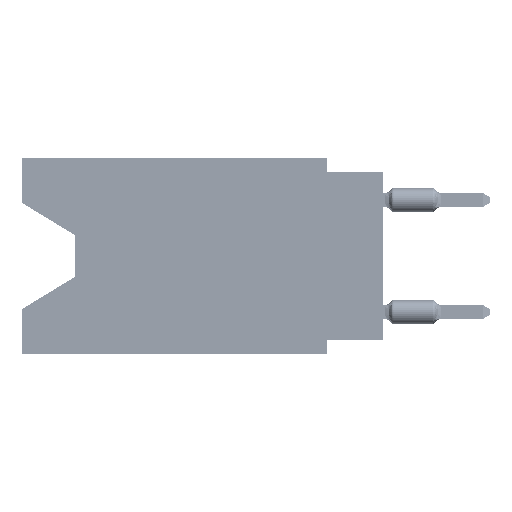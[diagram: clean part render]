
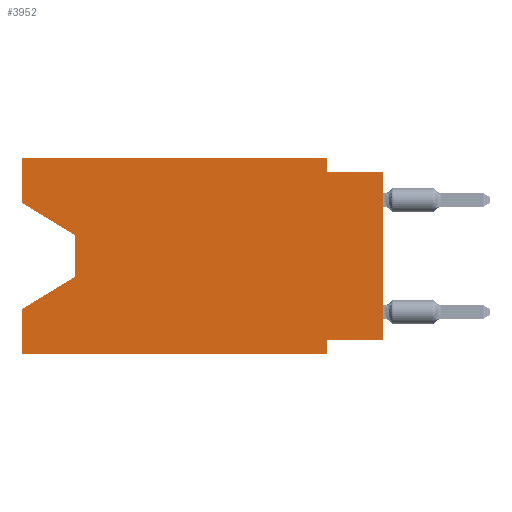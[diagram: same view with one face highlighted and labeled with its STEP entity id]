
A CAD part, left-side view. The second image highlights one B-rep face of the part: STEP entity #3952.
In plain terms, the highlighted planar face has unit normal (-1, 0, 0).
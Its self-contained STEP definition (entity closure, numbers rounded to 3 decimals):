
#749 = DIRECTION ( 'NONE',  ( 0., 0., 1. ) ) ;
#842 = VECTOR ( 'NONE', #63957, 1000. ) ;
#1870 = ORIENTED_EDGE ( 'NONE', *, *, #36977, .F. ) ;
#2698 = LINE ( 'NONE', #42277, #842 ) ;
#2990 = VECTOR ( 'NONE', #46452, 1000. ) ;
#3332 = VECTOR ( 'NONE', #9273, 1000. ) ;
#3509 = CARTESIAN_POINT ( 'NONE',  ( 0., 0., 0. ) ) ;
#3927 = EDGE_CURVE ( 'NONE', #44128, #29172, #12107, .T. ) ;
#3952 = ADVANCED_FACE ( 'NONE', ( #28903 ), #52056, .F. ) ;
#4749 = EDGE_CURVE ( 'NONE', #51776, #22948, #20185, .T. ) ;
#5682 = ORIENTED_EDGE ( 'NONE', *, *, #47351, .F. ) ;
#6222 = ORIENTED_EDGE ( 'NONE', *, *, #25716, .T. ) ;
#6600 = ORIENTED_EDGE ( 'NONE', *, *, #39897, .F. ) ;
#6983 = DIRECTION ( 'NONE',  ( 0., 1., 0. ) ) ;
#7105 = CARTESIAN_POINT ( 'NONE',  ( 0., 16.383, 0. ) ) ;
#7772 = VERTEX_POINT ( 'NONE', #64254 ) ;
#8877 = EDGE_CURVE ( 'NONE', #12186, #42481, #66267, .T. ) ;
#9273 = DIRECTION ( 'NONE',  ( 0., -0.855, -0.519 ) ) ;
#9658 = ORIENTED_EDGE ( 'NONE', *, *, #40314, .F. ) ;
#10961 = CARTESIAN_POINT ( 'NONE',  ( 0., 2.54, -0.635 ) ) ;
#11865 = DIRECTION ( 'NONE',  ( 0., -1., 0. ) ) ;
#12107 = LINE ( 'NONE', #68491, #2990 ) ;
#12186 = VERTEX_POINT ( 'NONE', #27859 ) ;
#12987 = VECTOR ( 'NONE', #15011, 1000. ) ;
#14540 = LINE ( 'NONE', #60436, #3332 ) ;
#15011 = DIRECTION ( 'NONE',  ( 0., 0., -1. ) ) ;
#15600 = ORIENTED_EDGE ( 'NONE', *, *, #35275, .T. ) ;
#17604 = CARTESIAN_POINT ( 'NONE',  ( 0., 13.97, -5.385 ) ) ;
#18115 = VECTOR ( 'NONE', #22621, 1000. ) ;
#18387 = CARTESIAN_POINT ( 'NONE',  ( 0., 0., -8.255 ) ) ;
#20185 = LINE ( 'NONE', #68590, #36137 ) ;
#20604 = CARTESIAN_POINT ( 'NONE',  ( 0., 13.97, -3.505 ) ) ;
#21716 = LINE ( 'NONE', #20604, #12987 ) ;
#22621 = DIRECTION ( 'NONE',  ( 0., 0., 1. ) ) ;
#22948 = VERTEX_POINT ( 'NONE', #38573 ) ;
#23405 = DIRECTION ( 'NONE',  ( 0., -1., 0. ) ) ;
#23709 = LINE ( 'NONE', #46496, #18115 ) ;
#24314 = VERTEX_POINT ( 'NONE', #18387 ) ;
#24667 = ORIENTED_EDGE ( 'NONE', *, *, #8877, .F. ) ;
#25716 = EDGE_CURVE ( 'NONE', #67044, #44128, #21716, .T. ) ;
#25722 = VECTOR ( 'NONE', #6983, 1000. ) ;
#26577 = VECTOR ( 'NONE', #11865, 1000. ) ;
#27199 = CARTESIAN_POINT ( 'NONE',  ( 0., 2.54, 0. ) ) ;
#27859 = CARTESIAN_POINT ( 'NONE',  ( 0., 16.383, 0. ) ) ;
#28168 = DIRECTION ( 'NONE',  ( 1., 0., 0. ) ) ;
#28249 = ORIENTED_EDGE ( 'NONE', *, *, #50553, .T. ) ;
#28538 = DIRECTION ( 'NONE',  ( 0., 0., -1. ) ) ;
#28903 = FACE_OUTER_BOUND ( 'NONE', #54279, .T. ) ;
#29172 = VERTEX_POINT ( 'NONE', #30144 ) ;
#29759 = LINE ( 'NONE', #68613, #25722 ) ;
#30144 = CARTESIAN_POINT ( 'NONE',  ( 0., 16.383, -6.852 ) ) ;
#35015 = CARTESIAN_POINT ( 'NONE',  ( 0., 2.54, -8.255 ) ) ;
#35275 = EDGE_CURVE ( 'NONE', #63538, #58508, #40969, .T. ) ;
#36137 = VECTOR ( 'NONE', #23405, 1000. ) ;
#36977 = EDGE_CURVE ( 'NONE', #42481, #51776, #66800, .T. ) ;
#37111 = VERTEX_POINT ( 'NONE', #35015 ) ;
#37740 = CARTESIAN_POINT ( 'NONE',  ( 0., 2.54, -8.89 ) ) ;
#38573 = CARTESIAN_POINT ( 'NONE',  ( 0., 0., -0.635 ) ) ;
#39369 = ORIENTED_EDGE ( 'NONE', *, *, #55566, .T. ) ;
#39897 = EDGE_CURVE ( 'NONE', #24314, #37111, #29759, .T. ) ;
#40314 = EDGE_CURVE ( 'NONE', #7772, #12186, #23709, .T. ) ;
#40969 = LINE ( 'NONE', #46199, #26577 ) ;
#41107 = ORIENTED_EDGE ( 'NONE', *, *, #3927, .T. ) ;
#42277 = CARTESIAN_POINT ( 'NONE',  ( 0., 2.54, -8.89 ) ) ;
#42481 = VERTEX_POINT ( 'NONE', #64257 ) ;
#44128 = VERTEX_POINT ( 'NONE', #17604 ) ;
#46199 = CARTESIAN_POINT ( 'NONE',  ( 0., 16.383, -8.89 ) ) ;
#46452 = DIRECTION ( 'NONE',  ( 0., 0.855, -0.519 ) ) ;
#46496 = CARTESIAN_POINT ( 'NONE',  ( 0., 16.383, 0. ) ) ;
#46568 = EDGE_CURVE ( 'NONE', #63538, #29172, #51921, .T. ) ;
#47351 = EDGE_CURVE ( 'NONE', #37111, #58508, #2698, .T. ) ;
#47432 = VECTOR ( 'NONE', #749, 1000. ) ;
#49064 = DIRECTION ( 'NONE',  ( 0., 0., 1. ) ) ;
#49105 = DIRECTION ( 'NONE',  ( 0., -1., 0. ) ) ;
#50525 = CARTESIAN_POINT ( 'NONE',  ( 0., 13.97, -3.505 ) ) ;
#50553 = EDGE_CURVE ( 'NONE', #7772, #67044, #14540, .T. ) ;
#50728 = DIRECTION ( 'NONE',  ( 0., 0., -1. ) ) ;
#51680 = CARTESIAN_POINT ( 'NONE',  ( 0., 16.383, 0. ) ) ;
#51776 = VERTEX_POINT ( 'NONE', #10961 ) ;
#51921 = LINE ( 'NONE', #7105, #47432 ) ;
#52056 = PLANE ( 'NONE',  #72133 ) ;
#54279 = EDGE_LOOP ( 'NONE', ( #28249, #6222, #41107, #57489, #15600, #5682, #6600, #39369, #59960, #1870, #24667, #9658 ) ) ;
#55566 = EDGE_CURVE ( 'NONE', #24314, #22948, #64776, .T. ) ;
#56196 = CARTESIAN_POINT ( 'NONE',  ( 0., 16.383, 0. ) ) ;
#57489 = ORIENTED_EDGE ( 'NONE', *, *, #46568, .F. ) ;
#57769 = VECTOR ( 'NONE', #50728, 1000. ) ;
#58508 = VERTEX_POINT ( 'NONE', #37740 ) ;
#59032 = VECTOR ( 'NONE', #49064, 1000. ) ;
#59960 = ORIENTED_EDGE ( 'NONE', *, *, #4749, .F. ) ;
#60436 = CARTESIAN_POINT ( 'NONE',  ( 0., 16.383, -2.038 ) ) ;
#62366 = VECTOR ( 'NONE', #49105, 1000. ) ;
#63538 = VERTEX_POINT ( 'NONE', #68909 ) ;
#63957 = DIRECTION ( 'NONE',  ( 0., 0., -1. ) ) ;
#64254 = CARTESIAN_POINT ( 'NONE',  ( 0., 16.383, -2.038 ) ) ;
#64257 = CARTESIAN_POINT ( 'NONE',  ( 0., 2.54, 0. ) ) ;
#64776 = LINE ( 'NONE', #3509, #59032 ) ;
#66267 = LINE ( 'NONE', #56196, #62366 ) ;
#66800 = LINE ( 'NONE', #27199, #57769 ) ;
#67044 = VERTEX_POINT ( 'NONE', #50525 ) ;
#68491 = CARTESIAN_POINT ( 'NONE',  ( 0., 13.97, -5.385 ) ) ;
#68590 = CARTESIAN_POINT ( 'NONE',  ( 0., 0., -0.635 ) ) ;
#68613 = CARTESIAN_POINT ( 'NONE',  ( 0., 0., -8.255 ) ) ;
#68909 = CARTESIAN_POINT ( 'NONE',  ( 0., 16.383, -8.89 ) ) ;
#72133 = AXIS2_PLACEMENT_3D ( 'NONE', #51680, #28168, #28538 ) ;
